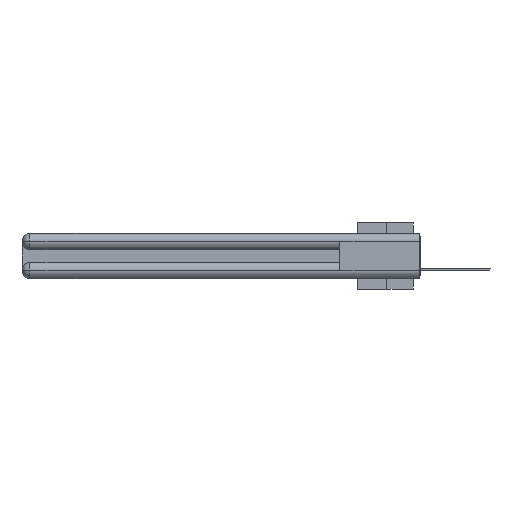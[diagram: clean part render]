
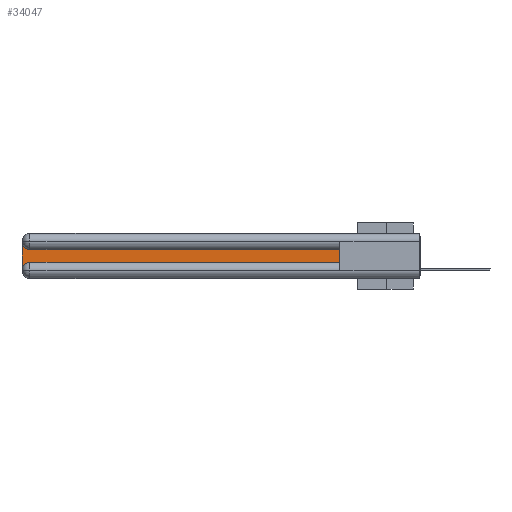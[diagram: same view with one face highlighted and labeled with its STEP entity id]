
A CAD part, left-side view. The second image highlights one B-rep face of the part: STEP entity #34047.
In plain terms, the highlighted planar face has unit normal (-1, 0, 0).
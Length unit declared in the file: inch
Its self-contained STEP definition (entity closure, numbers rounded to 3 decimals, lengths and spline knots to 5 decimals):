
#126 = VERTEX_POINT ( 'NONE', #17939 ) ;
#955 = CARTESIAN_POINT ( 'NONE',  ( 0.075, 0.6, -0.2175 ) ) ;
#1100 = DIRECTION ( 'NONE',  ( 0., 0., -1. ) ) ;
#1981 = VECTOR ( 'NONE', #12785, 39.37008 ) ;
#2078 = CARTESIAN_POINT ( 'NONE',  ( 0.075, 3., -0.0625 ) ) ;
#2858 = CARTESIAN_POINT ( 'NONE',  ( 0.075, 2.94, -0.1225 ) ) ;
#3341 = CARTESIAN_POINT ( 'NONE',  ( 0.075, 0.6, -0.2175 ) ) ;
#4192 = DIRECTION ( 'NONE',  ( 0., 0., -1. ) ) ;
#4310 = VERTEX_POINT ( 'NONE', #2858 ) ;
#4457 = CARTESIAN_POINT ( 'NONE',  ( 0.075, 2.94, -0.2175 ) ) ;
#5437 = VERTEX_POINT ( 'NONE', #4457 ) ;
#6051 = VERTEX_POINT ( 'NONE', #11578 ) ;
#6139 = VERTEX_POINT ( 'NONE', #13644 ) ;
#7154 = AXIS2_PLACEMENT_3D ( 'NONE', #9072, #32991, #1100 ) ;
#9048 = EDGE_CURVE ( 'NONE', #16232, #6051, #18536, .T. ) ;
#9056 = DIRECTION ( 'NONE',  ( 0., 0., -1. ) ) ;
#9072 = CARTESIAN_POINT ( 'NONE',  ( 0.075, 2.94, -0.0625 ) ) ;
#9118 = DIRECTION ( 'NONE',  ( 0., 0., 1. ) ) ;
#9463 = VECTOR ( 'NONE', #26158, 39.37008 ) ;
#9671 = CIRCLE ( 'NONE', #10344, 0.06 ) ;
#9708 = DIRECTION ( 'NONE',  ( 1., 0., 0. ) ) ;
#9823 = PLANE ( 'NONE',  #19333 ) ;
#10344 = AXIS2_PLACEMENT_3D ( 'NONE', #32852, #32747, #9056 ) ;
#11355 = ORIENTED_EDGE ( 'NONE', *, *, #9048, .T. ) ;
#11403 = FACE_OUTER_BOUND ( 'NONE', #21780, .T. ) ;
#11578 = CARTESIAN_POINT ( 'NONE',  ( 0.075, 3., -0.2775 ) ) ;
#12051 = ORIENTED_EDGE ( 'NONE', *, *, #32936, .T. ) ;
#12702 = ORIENTED_EDGE ( 'NONE', *, *, #27754, .T. ) ;
#12785 = DIRECTION ( 'NONE',  ( 0., 1., 0. ) ) ;
#13644 = CARTESIAN_POINT ( 'NONE',  ( 0.075, 0.6, -0.2175 ) ) ;
#14361 = LINE ( 'NONE', #26548, #1981 ) ;
#15924 = EDGE_CURVE ( 'NONE', #6139, #126, #18066, .T. ) ;
#16232 = VERTEX_POINT ( 'NONE', #2078 ) ;
#17180 = CARTESIAN_POINT ( 'NONE',  ( 0.075, 3., -0.2175 ) ) ;
#17725 = ORIENTED_EDGE ( 'NONE', *, *, #15924, .T. ) ;
#17939 = CARTESIAN_POINT ( 'NONE',  ( 0.075, 0.6, -0.1225 ) ) ;
#18066 = LINE ( 'NONE', #3341, #28430 ) ;
#18536 = LINE ( 'NONE', #17180, #9463 ) ;
#19333 = AXIS2_PLACEMENT_3D ( 'NONE', #33517, #9708, #4192 ) ;
#21780 = EDGE_LOOP ( 'NONE', ( #12051, #29268, #11355, #12702, #25555, #17725 ) ) ;
#22601 = VECTOR ( 'NONE', #24669, 39.37008 ) ;
#22982 = EDGE_CURVE ( 'NONE', #4310, #16232, #23232, .T. ) ;
#23232 = CIRCLE ( 'NONE', #7154, 0.06 ) ;
#24267 = LINE ( 'NONE', #955, #22601 ) ;
#24669 = DIRECTION ( 'NONE',  ( 0., -1., 0. ) ) ;
#25555 = ORIENTED_EDGE ( 'NONE', *, *, #26040, .T. ) ;
#26040 = EDGE_CURVE ( 'NONE', #5437, #6139, #24267, .T. ) ;
#26158 = DIRECTION ( 'NONE',  ( 0., 0., -1. ) ) ;
#26548 = CARTESIAN_POINT ( 'NONE',  ( 0.075, 0.6, -0.1225 ) ) ;
#27754 = EDGE_CURVE ( 'NONE', #6051, #5437, #9671, .T. ) ;
#28430 = VECTOR ( 'NONE', #9118, 39.37008 ) ;
#29268 = ORIENTED_EDGE ( 'NONE', *, *, #22982, .T. ) ;
#32747 = DIRECTION ( 'NONE',  ( 1., 0., 0. ) ) ;
#32852 = CARTESIAN_POINT ( 'NONE',  ( 0.075, 2.94, -0.2775 ) ) ;
#32936 = EDGE_CURVE ( 'NONE', #126, #4310, #14361, .T. ) ;
#32991 = DIRECTION ( 'NONE',  ( 1., 0., 0. ) ) ;
#33517 = CARTESIAN_POINT ( 'NONE',  ( 0.075, 3., -0.1225 ) ) ;
#34047 = ADVANCED_FACE ( 'NONE', ( #11403 ), #9823, .F. ) ;
